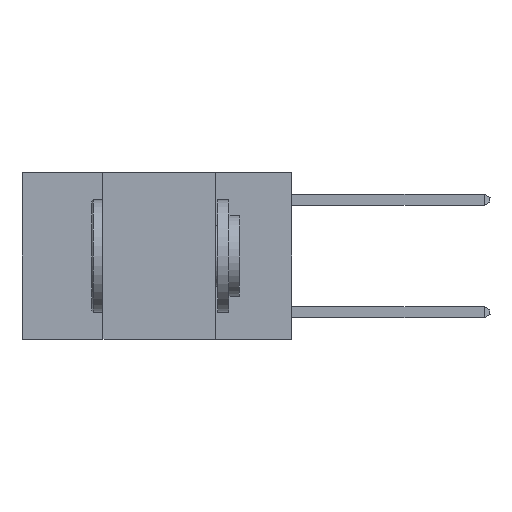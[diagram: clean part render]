
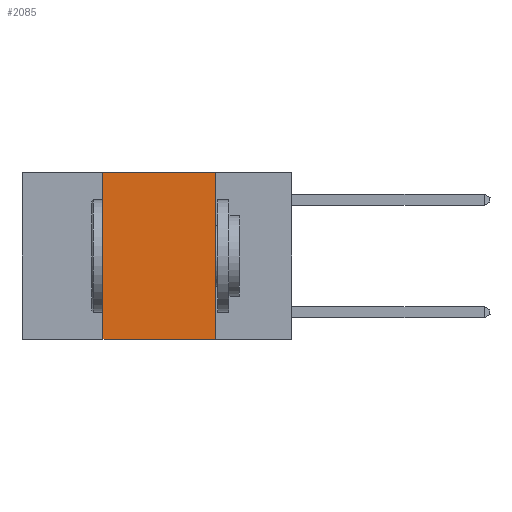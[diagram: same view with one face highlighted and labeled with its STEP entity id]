
A CAD part, left-side view. The second image highlights one B-rep face of the part: STEP entity #2085.
In plain terms, the highlighted planar face has unit normal (-1, 0, 0).
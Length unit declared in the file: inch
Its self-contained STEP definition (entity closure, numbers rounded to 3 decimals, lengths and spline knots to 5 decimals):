
#317 = FACE_OUTER_BOUND ( 'NONE', #23503, .T. ) ;
#676 = CARTESIAN_POINT ( 'NONE',  ( 0., 0.17, 0. ) ) ;
#794 = VECTOR ( 'NONE', #17602, 39.37008 ) ;
#1310 = VERTEX_POINT ( 'NONE', #20408 ) ;
#2085 = ADVANCED_FACE ( 'NONE', ( #317 ), #21070, .F. ) ;
#3864 = CARTESIAN_POINT ( 'NONE',  ( 0., 0.6, 0. ) ) ;
#5544 = ORIENTED_EDGE ( 'NONE', *, *, #12256, .F. ) ;
#5587 = VERTEX_POINT ( 'NONE', #16979 ) ;
#8281 = VECTOR ( 'NONE', #15327, 39.37008 ) ;
#8929 = EDGE_CURVE ( 'NONE', #1310, #12259, #11488, .T. ) ;
#9238 = CARTESIAN_POINT ( 'NONE',  ( 0., 0.42, 0. ) ) ;
#11488 = LINE ( 'NONE', #9238, #18494 ) ;
#11493 = VECTOR ( 'NONE', #13145, 39.37008 ) ;
#11813 = DIRECTION ( 'NONE',  ( 1., 0., 0. ) ) ;
#12256 = EDGE_CURVE ( 'NONE', #15057, #5587, #19688, .T. ) ;
#12259 = VERTEX_POINT ( 'NONE', #21544 ) ;
#12422 = AXIS2_PLACEMENT_3D ( 'NONE', #19241, #11813, #17247 ) ;
#12911 = LINE ( 'NONE', #3864, #11493 ) ;
#13145 = DIRECTION ( 'NONE',  ( 0., -1., 0. ) ) ;
#14852 = EDGE_CURVE ( 'NONE', #1310, #5587, #15690, .T. ) ;
#15057 = VERTEX_POINT ( 'NONE', #16646 ) ;
#15327 = DIRECTION ( 'NONE',  ( 0., -1., 0. ) ) ;
#15690 = LINE ( 'NONE', #23216, #8281 ) ;
#16388 = ORIENTED_EDGE ( 'NONE', *, *, #8929, .F. ) ;
#16553 = EDGE_CURVE ( 'NONE', #12259, #15057, #12911, .T. ) ;
#16646 = CARTESIAN_POINT ( 'NONE',  ( 0., 0.17, 0. ) ) ;
#16823 = DIRECTION ( 'NONE',  ( 0., 0., 1. ) ) ;
#16979 = CARTESIAN_POINT ( 'NONE',  ( 0., 0.17, -0.37 ) ) ;
#17247 = DIRECTION ( 'NONE',  ( 0., 0., -1. ) ) ;
#17602 = DIRECTION ( 'NONE',  ( 0., 0., -1. ) ) ;
#18110 = ORIENTED_EDGE ( 'NONE', *, *, #14852, .T. ) ;
#18494 = VECTOR ( 'NONE', #16823, 39.37008 ) ;
#19241 = CARTESIAN_POINT ( 'NONE',  ( 0., 0.6, 0. ) ) ;
#19688 = LINE ( 'NONE', #676, #794 ) ;
#20408 = CARTESIAN_POINT ( 'NONE',  ( 0., 0.42, -0.37 ) ) ;
#21070 = PLANE ( 'NONE',  #12422 ) ;
#21544 = CARTESIAN_POINT ( 'NONE',  ( 0., 0.42, 0. ) ) ;
#23203 = ORIENTED_EDGE ( 'NONE', *, *, #16553, .F. ) ;
#23216 = CARTESIAN_POINT ( 'NONE',  ( 0., 0.6, -0.37 ) ) ;
#23503 = EDGE_LOOP ( 'NONE', ( #5544, #23203, #16388, #18110 ) ) ;
